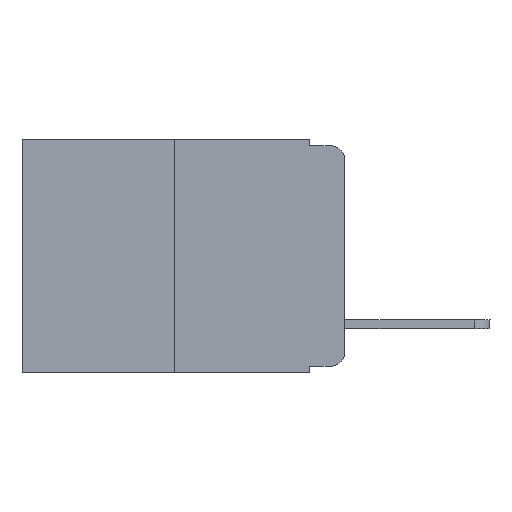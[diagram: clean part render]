
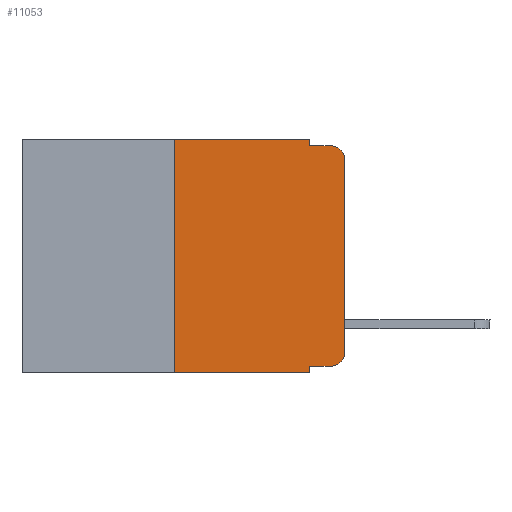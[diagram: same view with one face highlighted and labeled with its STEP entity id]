
A CAD part, left-side view. The second image highlights one B-rep face of the part: STEP entity #11053.
In plain terms, the highlighted planar face has unit normal (-1, 0, 0).
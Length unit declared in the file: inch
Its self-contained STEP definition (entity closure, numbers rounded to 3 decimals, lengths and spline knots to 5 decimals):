
#172 = VECTOR ( 'NONE', #12758, 39.37008 ) ;
#356 = LINE ( 'NONE', #15859, #172 ) ;
#529 = CARTESIAN_POINT ( 'NONE',  ( 0., 0., 0. ) ) ;
#578 = DIRECTION ( 'NONE',  ( 0., 0., -1. ) ) ;
#664 = CARTESIAN_POINT ( 'NONE',  ( 0., 0.02, -0.03 ) ) ;
#726 = DIRECTION ( 'NONE',  ( -1., 0., 0. ) ) ;
#891 = PLANE ( 'NONE',  #2493 ) ;
#1341 = EDGE_CURVE ( 'NONE', #10934, #12015, #6347, .T. ) ;
#1487 = DIRECTION ( 'NONE',  ( 0., 0., -1. ) ) ;
#1627 = LINE ( 'NONE', #15766, #14901 ) ;
#2491 = ORIENTED_EDGE ( 'NONE', *, *, #16363, .T. ) ;
#2493 = AXIS2_PLACEMENT_3D ( 'NONE', #10583, #6228, #10763 ) ;
#2572 = EDGE_CURVE ( 'NONE', #8603, #5661, #4704, .T. ) ;
#2685 = CIRCLE ( 'NONE', #11439, 0.02 ) ;
#2984 = DIRECTION ( 'NONE',  ( 0., -1., 0. ) ) ;
#3466 = FACE_OUTER_BOUND ( 'NONE', #10299, .T. ) ;
#3509 = EDGE_CURVE ( 'NONE', #4475, #12033, #15930, .T. ) ;
#3646 = VECTOR ( 'NONE', #2984, 39.37008 ) ;
#4088 = LINE ( 'NONE', #11085, #3646 ) ;
#4397 = CARTESIAN_POINT ( 'NONE',  ( 0., 0., -0.313 ) ) ;
#4475 = VERTEX_POINT ( 'NONE', #9856 ) ;
#4666 = EDGE_CURVE ( 'NONE', #5182, #13987, #1627, .T. ) ;
#4704 = LINE ( 'NONE', #10340, #11849 ) ;
#4917 = LINE ( 'NONE', #10634, #10115 ) ;
#5069 = EDGE_CURVE ( 'NONE', #15582, #12033, #2685, .T. ) ;
#5182 = VERTEX_POINT ( 'NONE', #7722 ) ;
#5661 = VERTEX_POINT ( 'NONE', #14103 ) ;
#6228 = DIRECTION ( 'NONE',  ( 1., 0., 0. ) ) ;
#6232 = AXIS2_PLACEMENT_3D ( 'NONE', #14251, #726, #1487 ) ;
#6347 = CIRCLE ( 'NONE', #6232, 0.02 ) ;
#6444 = ORIENTED_EDGE ( 'NONE', *, *, #12324, .F. ) ;
#6477 = ORIENTED_EDGE ( 'NONE', *, *, #9948, .T. ) ;
#6675 = LINE ( 'NONE', #14571, #8929 ) ;
#6776 = CARTESIAN_POINT ( 'NONE',  ( 0., 0.051, -0.333 ) ) ;
#7310 = VECTOR ( 'NONE', #11646, 39.37008 ) ;
#7722 = CARTESIAN_POINT ( 'NONE',  ( 0., 0.25, -0.343 ) ) ;
#7820 = CARTESIAN_POINT ( 'NONE',  ( 0., 0.25, 0. ) ) ;
#8603 = VERTEX_POINT ( 'NONE', #6776 ) ;
#8929 = VECTOR ( 'NONE', #13211, 39.37008 ) ;
#9254 = CARTESIAN_POINT ( 'NONE',  ( 0., 0., -0.03 ) ) ;
#9856 = CARTESIAN_POINT ( 'NONE',  ( 0., 0.051, -0.01 ) ) ;
#9948 = EDGE_CURVE ( 'NONE', #5182, #5661, #4088, .T. ) ;
#10115 = VECTOR ( 'NONE', #14355, 39.37008 ) ;
#10299 = EDGE_LOOP ( 'NONE', ( #2491, #10648, #13914, #13439, #6444, #15148, #6477, #14606, #12120, #15786 ) ) ;
#10340 = CARTESIAN_POINT ( 'NONE',  ( 0., 0.051, 0. ) ) ;
#10583 = CARTESIAN_POINT ( 'NONE',  ( 0., 0.473, 0. ) ) ;
#10634 = CARTESIAN_POINT ( 'NONE',  ( 0., 0.051, 0. ) ) ;
#10648 = ORIENTED_EDGE ( 'NONE', *, *, #5069, .T. ) ;
#10763 = DIRECTION ( 'NONE',  ( 0., 0., -1. ) ) ;
#10799 = VERTEX_POINT ( 'NONE', #13674 ) ;
#10914 = EDGE_CURVE ( 'NONE', #8603, #10934, #356, .T. ) ;
#10934 = VERTEX_POINT ( 'NONE', #14477 ) ;
#11053 = ADVANCED_FACE ( 'NONE', ( #3466 ), #891, .F. ) ;
#11085 = CARTESIAN_POINT ( 'NONE',  ( 0., 0.473, -0.343 ) ) ;
#11128 = CARTESIAN_POINT ( 'NONE',  ( 0., 0.02, -0.01 ) ) ;
#11300 = DIRECTION ( 'NONE',  ( 0., 0., 1. ) ) ;
#11439 = AXIS2_PLACEMENT_3D ( 'NONE', #664, #13252, #578 ) ;
#11646 = DIRECTION ( 'NONE',  ( 0., -1., 0. ) ) ;
#11849 = VECTOR ( 'NONE', #13160, 39.37008 ) ;
#12015 = VERTEX_POINT ( 'NONE', #4397 ) ;
#12033 = VERTEX_POINT ( 'NONE', #11128 ) ;
#12120 = ORIENTED_EDGE ( 'NONE', *, *, #10914, .T. ) ;
#12324 = EDGE_CURVE ( 'NONE', #13987, #10799, #6675, .T. ) ;
#12758 = DIRECTION ( 'NONE',  ( 0., -1., 0. ) ) ;
#13016 = LINE ( 'NONE', #529, #13867 ) ;
#13160 = DIRECTION ( 'NONE',  ( 0., 0., -1. ) ) ;
#13211 = DIRECTION ( 'NONE',  ( 0., -1., 0. ) ) ;
#13252 = DIRECTION ( 'NONE',  ( -1., 0., 0. ) ) ;
#13439 = ORIENTED_EDGE ( 'NONE', *, *, #16924, .F. ) ;
#13674 = CARTESIAN_POINT ( 'NONE',  ( 0., 0.051, 0. ) ) ;
#13867 = VECTOR ( 'NONE', #11300, 39.37008 ) ;
#13914 = ORIENTED_EDGE ( 'NONE', *, *, #3509, .F. ) ;
#13987 = VERTEX_POINT ( 'NONE', #7820 ) ;
#14103 = CARTESIAN_POINT ( 'NONE',  ( 0., 0.051, -0.343 ) ) ;
#14251 = CARTESIAN_POINT ( 'NONE',  ( 0., 0.02, -0.313 ) ) ;
#14355 = DIRECTION ( 'NONE',  ( 0., 0., -1. ) ) ;
#14449 = CARTESIAN_POINT ( 'NONE',  ( 0., 0.051, -0.01 ) ) ;
#14477 = CARTESIAN_POINT ( 'NONE',  ( 0., 0.02, -0.333 ) ) ;
#14571 = CARTESIAN_POINT ( 'NONE',  ( 0., 0.473, 0. ) ) ;
#14606 = ORIENTED_EDGE ( 'NONE', *, *, #2572, .F. ) ;
#14901 = VECTOR ( 'NONE', #15678, 39.37008 ) ;
#15148 = ORIENTED_EDGE ( 'NONE', *, *, #4666, .F. ) ;
#15582 = VERTEX_POINT ( 'NONE', #9254 ) ;
#15678 = DIRECTION ( 'NONE',  ( 0., 0., 1. ) ) ;
#15766 = CARTESIAN_POINT ( 'NONE',  ( 0., 0.25, 0. ) ) ;
#15786 = ORIENTED_EDGE ( 'NONE', *, *, #1341, .T. ) ;
#15859 = CARTESIAN_POINT ( 'NONE',  ( 0., 0.051, -0.333 ) ) ;
#15930 = LINE ( 'NONE', #14449, #7310 ) ;
#16363 = EDGE_CURVE ( 'NONE', #12015, #15582, #13016, .T. ) ;
#16924 = EDGE_CURVE ( 'NONE', #10799, #4475, #4917, .T. ) ;
